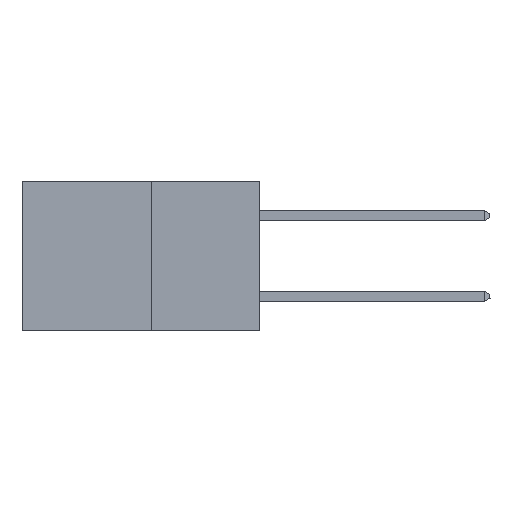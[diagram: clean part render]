
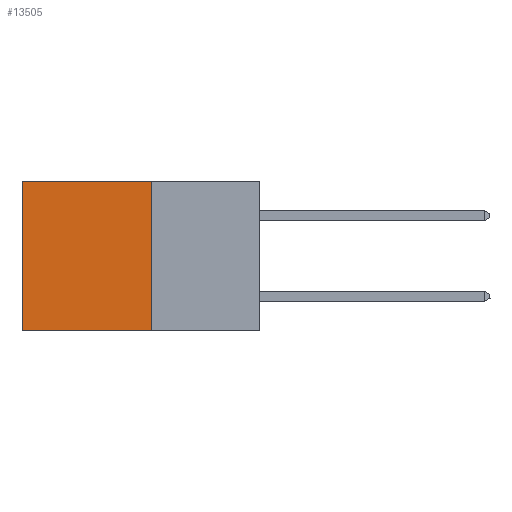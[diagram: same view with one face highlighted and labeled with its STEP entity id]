
A CAD part, left-side view. The second image highlights one B-rep face of the part: STEP entity #13505.
In plain terms, the highlighted planar face has unit normal (-1, 0, 0).
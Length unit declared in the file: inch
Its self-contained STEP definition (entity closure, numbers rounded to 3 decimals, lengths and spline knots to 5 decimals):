
#473 = LINE ( 'NONE', #24549, #6729 ) ;
#1805 = CARTESIAN_POINT ( 'NONE',  ( 0.277, 0.59, -0.37 ) ) ;
#1936 = VERTEX_POINT ( 'NONE', #27037 ) ;
#2783 = CARTESIAN_POINT ( 'NONE',  ( 0.277, 0.27, -0.37 ) ) ;
#2795 = EDGE_CURVE ( 'NONE', #1936, #28322, #14427, .T. ) ;
#5142 = DIRECTION ( 'NONE',  ( 0., 0., -1. ) ) ;
#5568 = DIRECTION ( 'NONE',  ( 0., 0., -1. ) ) ;
#5734 = CARTESIAN_POINT ( 'NONE',  ( 0.277, 0.27, -0.37 ) ) ;
#6463 = EDGE_CURVE ( 'NONE', #1936, #12082, #7618, .T. ) ;
#6729 = VECTOR ( 'NONE', #8956, 39.37008 ) ;
#6825 = CARTESIAN_POINT ( 'NONE',  ( 0.277, 0.59, -0.37 ) ) ;
#7415 = ORIENTED_EDGE ( 'NONE', *, *, #2795, .T. ) ;
#7618 = LINE ( 'NONE', #5734, #24737 ) ;
#8442 = DIRECTION ( 'NONE',  ( 0., 1., 0. ) ) ;
#8548 = LINE ( 'NONE', #6825, #19787 ) ;
#8956 = DIRECTION ( 'NONE',  ( 0., 1., 0. ) ) ;
#9962 = EDGE_CURVE ( 'NONE', #12082, #28748, #473, .T. ) ;
#11100 = FACE_OUTER_BOUND ( 'NONE', #25934, .T. ) ;
#12082 = VERTEX_POINT ( 'NONE', #20497 ) ;
#13505 = ADVANCED_FACE ( 'NONE', ( #11100 ), #25255, .F. ) ;
#13998 = ORIENTED_EDGE ( 'NONE', *, *, #14735, .T. ) ;
#14427 = LINE ( 'NONE', #20219, #25878 ) ;
#14735 = EDGE_CURVE ( 'NONE', #28322, #28748, #8548, .T. ) ;
#16502 = CARTESIAN_POINT ( 'NONE',  ( 0.277, 0.59, 0. ) ) ;
#18145 = ORIENTED_EDGE ( 'NONE', *, *, #9962, .F. ) ;
#18704 = DIRECTION ( 'NONE',  ( 1., 0., 0. ) ) ;
#18907 = ORIENTED_EDGE ( 'NONE', *, *, #6463, .F. ) ;
#19787 = VECTOR ( 'NONE', #20312, 39.37008 ) ;
#20219 = CARTESIAN_POINT ( 'NONE',  ( 0.277, 0.27, 0. ) ) ;
#20312 = DIRECTION ( 'NONE',  ( 0., 0., -1. ) ) ;
#20497 = CARTESIAN_POINT ( 'NONE',  ( 0.277, 0.27, -0.37 ) ) ;
#24549 = CARTESIAN_POINT ( 'NONE',  ( 0.277, 0.27, -0.37 ) ) ;
#24737 = VECTOR ( 'NONE', #5568, 39.37008 ) ;
#25255 = PLANE ( 'NONE',  #26307 ) ;
#25878 = VECTOR ( 'NONE', #8442, 39.37008 ) ;
#25934 = EDGE_LOOP ( 'NONE', ( #13998, #18145, #18907, #7415 ) ) ;
#26307 = AXIS2_PLACEMENT_3D ( 'NONE', #2783, #18704, #5142 ) ;
#27037 = CARTESIAN_POINT ( 'NONE',  ( 0.277, 0.27, 0. ) ) ;
#28322 = VERTEX_POINT ( 'NONE', #16502 ) ;
#28748 = VERTEX_POINT ( 'NONE', #1805 ) ;
